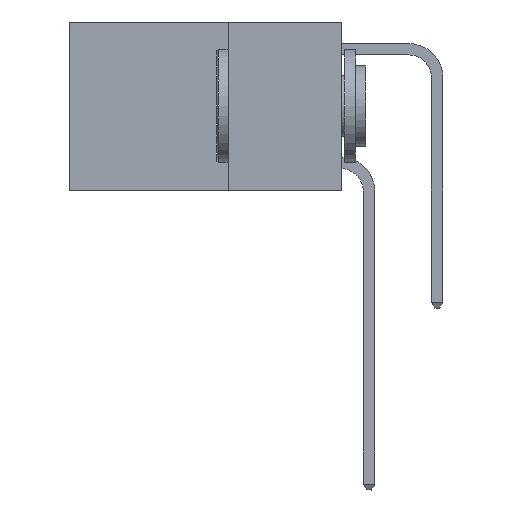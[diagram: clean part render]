
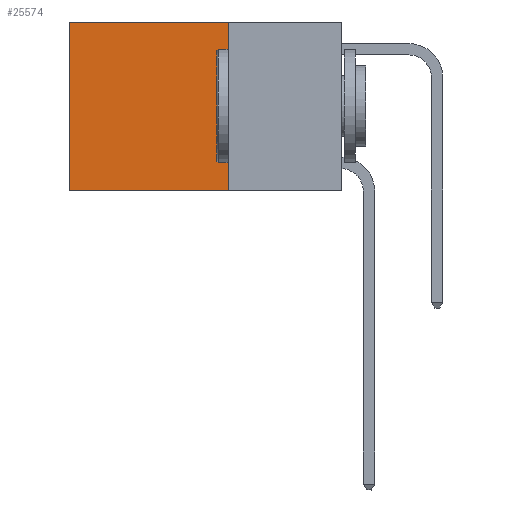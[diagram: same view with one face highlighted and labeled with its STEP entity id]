
A CAD part, left-side view. The second image highlights one B-rep face of the part: STEP entity #25574.
In plain terms, the highlighted planar face has unit normal (-1, 0, 0).
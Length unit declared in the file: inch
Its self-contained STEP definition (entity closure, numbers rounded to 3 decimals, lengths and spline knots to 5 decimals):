
#2174 = ORIENTED_EDGE ( 'NONE', *, *, #17190, .F. ) ;
#2587 = LINE ( 'NONE', #7703, #22112 ) ;
#4104 = AXIS2_PLACEMENT_3D ( 'NONE', #13209, #27179, #15816 ) ;
#4667 = VECTOR ( 'NONE', #17049, 39.37008 ) ;
#6257 = LINE ( 'NONE', #28798, #13496 ) ;
#7497 = CARTESIAN_POINT ( 'NONE',  ( 0.2625, 0.25, -0.37 ) ) ;
#7703 = CARTESIAN_POINT ( 'NONE',  ( 0.2625, 0.25, 0. ) ) ;
#7788 = CARTESIAN_POINT ( 'NONE',  ( 0.2625, 0.25, 0. ) ) ;
#8928 = VECTOR ( 'NONE', #20636, 39.37008 ) ;
#10041 = EDGE_CURVE ( 'NONE', #21739, #22218, #2587, .T. ) ;
#10047 = VERTEX_POINT ( 'NONE', #7497 ) ;
#11142 = CARTESIAN_POINT ( 'NONE',  ( 0.2625, 0.25, 0. ) ) ;
#11550 = EDGE_CURVE ( 'NONE', #22218, #19073, #23854, .T. ) ;
#13209 = CARTESIAN_POINT ( 'NONE',  ( 0.2625, 0.25, 0. ) ) ;
#13496 = VECTOR ( 'NONE', #24353, 39.37008 ) ;
#14358 = LINE ( 'NONE', #11142, #8928 ) ;
#14556 = ORIENTED_EDGE ( 'NONE', *, *, #10041, .T. ) ;
#14887 = CARTESIAN_POINT ( 'NONE',  ( 0.2625, 0.6, 0. ) ) ;
#15816 = DIRECTION ( 'NONE',  ( 0., 0., -1. ) ) ;
#17049 = DIRECTION ( 'NONE',  ( 0., 0., -1. ) ) ;
#17190 = EDGE_CURVE ( 'NONE', #10047, #19073, #6257, .T. ) ;
#17973 = FACE_OUTER_BOUND ( 'NONE', #20275, .T. ) ;
#18083 = ORIENTED_EDGE ( 'NONE', *, *, #11550, .T. ) ;
#19073 = VERTEX_POINT ( 'NONE', #27382 ) ;
#20275 = EDGE_LOOP ( 'NONE', ( #18083, #2174, #29717, #14556 ) ) ;
#20636 = DIRECTION ( 'NONE',  ( 0., 0., -1. ) ) ;
#21739 = VERTEX_POINT ( 'NONE', #7788 ) ;
#22112 = VECTOR ( 'NONE', #23776, 39.37008 ) ;
#22218 = VERTEX_POINT ( 'NONE', #26750 ) ;
#22617 = PLANE ( 'NONE',  #4104 ) ;
#23776 = DIRECTION ( 'NONE',  ( 0., 1., 0. ) ) ;
#23854 = LINE ( 'NONE', #14887, #4667 ) ;
#24353 = DIRECTION ( 'NONE',  ( 0., 1., 0. ) ) ;
#25367 = EDGE_CURVE ( 'NONE', #21739, #10047, #14358, .T. ) ;
#25574 = ADVANCED_FACE ( 'NONE', ( #17973 ), #22617, .F. ) ;
#26750 = CARTESIAN_POINT ( 'NONE',  ( 0.2625, 0.6, 0. ) ) ;
#27179 = DIRECTION ( 'NONE',  ( 1., 0., 0. ) ) ;
#27382 = CARTESIAN_POINT ( 'NONE',  ( 0.2625, 0.6, -0.37 ) ) ;
#28798 = CARTESIAN_POINT ( 'NONE',  ( 0.2625, 0.25, -0.37 ) ) ;
#29717 = ORIENTED_EDGE ( 'NONE', *, *, #25367, .F. ) ;
